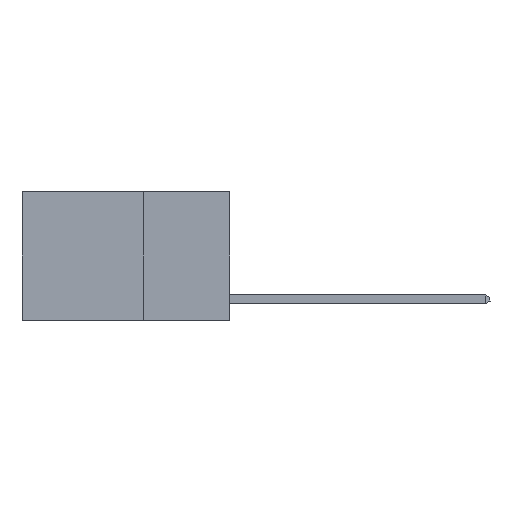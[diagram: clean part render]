
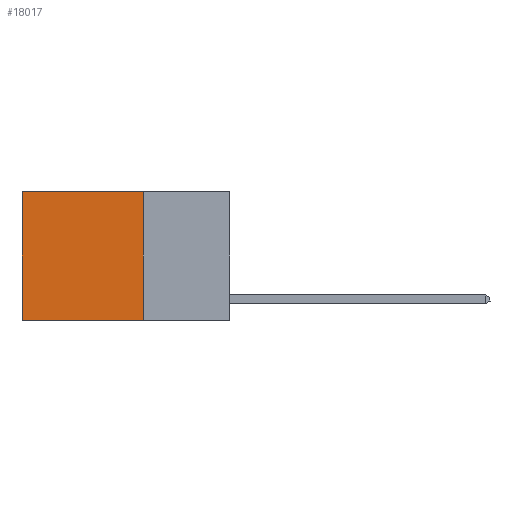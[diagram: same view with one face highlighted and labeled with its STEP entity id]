
A CAD part, left-side view. The second image highlights one B-rep face of the part: STEP entity #18017.
In plain terms, the highlighted planar face has unit normal (-1, 0, 0).
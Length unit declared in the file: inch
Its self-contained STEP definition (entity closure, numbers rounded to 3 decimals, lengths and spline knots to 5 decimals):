
#1252 = ORIENTED_EDGE ( 'NONE', *, *, #9040, .T. ) ;
#1582 = DIRECTION ( 'NONE',  ( 0., 1., 0. ) ) ;
#1651 = CARTESIAN_POINT ( 'NONE',  ( 0.2625, 0.25, 0. ) ) ;
#1669 = ORIENTED_EDGE ( 'NONE', *, *, #5180, .T. ) ;
#2011 = VECTOR ( 'NONE', #1582, 39.37008 ) ;
#2533 = DIRECTION ( 'NONE',  ( 1., 0., 0. ) ) ;
#2536 = VERTEX_POINT ( 'NONE', #9064 ) ;
#3691 = VECTOR ( 'NONE', #17593, 39.37008 ) ;
#4627 = CARTESIAN_POINT ( 'NONE',  ( 0.2625, 0.25, -0.37 ) ) ;
#4733 = VECTOR ( 'NONE', #11776, 39.37008 ) ;
#4756 = FACE_OUTER_BOUND ( 'NONE', #13002, .T. ) ;
#5180 = EDGE_CURVE ( 'NONE', #6564, #2536, #8921, .T. ) ;
#6564 = VERTEX_POINT ( 'NONE', #13503 ) ;
#6643 = CARTESIAN_POINT ( 'NONE',  ( 0.2625, 0.25, 0. ) ) ;
#7104 = CARTESIAN_POINT ( 'NONE',  ( 0.2625, 0.25, -0.37 ) ) ;
#7240 = PLANE ( 'NONE',  #14029 ) ;
#7870 = LINE ( 'NONE', #6643, #3691 ) ;
#8107 = ORIENTED_EDGE ( 'NONE', *, *, #20302, .F. ) ;
#8921 = LINE ( 'NONE', #17895, #4733 ) ;
#9040 = EDGE_CURVE ( 'NONE', #9686, #6564, #10517, .T. ) ;
#9064 = CARTESIAN_POINT ( 'NONE',  ( 0.2625, 0.6, -0.37 ) ) ;
#9686 = VERTEX_POINT ( 'NONE', #12465 ) ;
#10371 = LINE ( 'NONE', #7104, #14038 ) ;
#10517 = LINE ( 'NONE', #1651, #2011 ) ;
#11776 = DIRECTION ( 'NONE',  ( 0., 0., -1. ) ) ;
#12065 = CARTESIAN_POINT ( 'NONE',  ( 0.2625, 0.25, 0. ) ) ;
#12465 = CARTESIAN_POINT ( 'NONE',  ( 0.2625, 0.25, 0. ) ) ;
#13002 = EDGE_LOOP ( 'NONE', ( #1669, #13874, #8107, #1252 ) ) ;
#13142 = EDGE_CURVE ( 'NONE', #16313, #2536, #10371, .T. ) ;
#13503 = CARTESIAN_POINT ( 'NONE',  ( 0.2625, 0.6, 0. ) ) ;
#13652 = DIRECTION ( 'NONE',  ( 0., 0., -1. ) ) ;
#13874 = ORIENTED_EDGE ( 'NONE', *, *, #13142, .F. ) ;
#14029 = AXIS2_PLACEMENT_3D ( 'NONE', #12065, #2533, #13652 ) ;
#14038 = VECTOR ( 'NONE', #19620, 39.37008 ) ;
#16313 = VERTEX_POINT ( 'NONE', #4627 ) ;
#17593 = DIRECTION ( 'NONE',  ( 0., 0., -1. ) ) ;
#17895 = CARTESIAN_POINT ( 'NONE',  ( 0.2625, 0.6, 0. ) ) ;
#18017 = ADVANCED_FACE ( 'NONE', ( #4756 ), #7240, .F. ) ;
#19620 = DIRECTION ( 'NONE',  ( 0., 1., 0. ) ) ;
#20302 = EDGE_CURVE ( 'NONE', #9686, #16313, #7870, .T. ) ;
